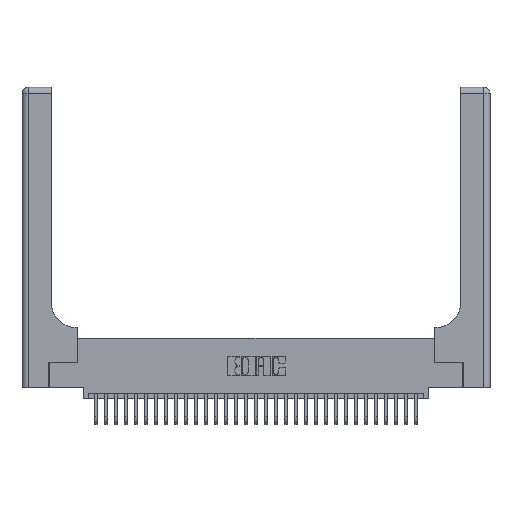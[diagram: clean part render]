
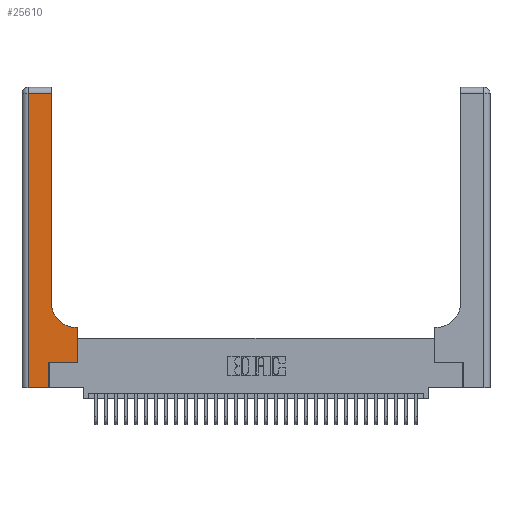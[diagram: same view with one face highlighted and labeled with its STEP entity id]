
A CAD part, top view. The second image highlights one B-rep face of the part: STEP entity #25610.
In plain terms, the highlighted planar face has unit normal (0, 0, 1).
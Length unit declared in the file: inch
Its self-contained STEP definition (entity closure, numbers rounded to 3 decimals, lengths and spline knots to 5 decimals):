
#931 = CARTESIAN_POINT ( 'NONE',  ( 0.269, 0.25, 0.37 ) ) ;
#1385 = VERTEX_POINT ( 'NONE', #3543 ) ;
#1602 = DIRECTION ( 'NONE',  ( 0., 1., 0. ) ) ;
#3370 = VECTOR ( 'NONE', #5774, 39.37008 ) ;
#3408 = CARTESIAN_POINT ( 'NONE',  ( 0.06, 3., 0.37 ) ) ;
#3427 = CARTESIAN_POINT ( 'NONE',  ( 0.06, 2.94, 0.37 ) ) ;
#3543 = CARTESIAN_POINT ( 'NONE',  ( 0.06, 0., 0.37 ) ) ;
#4092 = CARTESIAN_POINT ( 'NONE',  ( 0., 2.94, 0.37 ) ) ;
#4132 = LINE ( 'NONE', #20401, #3370 ) ;
#4817 = DIRECTION ( 'NONE',  ( 1., 0., 0. ) ) ;
#5692 = AXIS2_PLACEMENT_3D ( 'NONE', #26367, #11873, #28790 ) ;
#5774 = DIRECTION ( 'NONE',  ( 0., 1., 0. ) ) ;
#6044 = ORIENTED_EDGE ( 'NONE', *, *, #14439, .T. ) ;
#6551 = DIRECTION ( 'NONE',  ( -1., 0., 0. ) ) ;
#6573 = EDGE_CURVE ( 'NONE', #22003, #24052, #29202, .T. ) ;
#7005 = CARTESIAN_POINT ( 'NONE',  ( 0.5585, 0.6, 0.37 ) ) ;
#7516 = VECTOR ( 'NONE', #29604, 39.37008 ) ;
#8048 = DIRECTION ( 'NONE',  ( 0., 1., 0. ) ) ;
#8100 = VERTEX_POINT ( 'NONE', #19926 ) ;
#8304 = DIRECTION ( 'NONE',  ( 0., -1., 0. ) ) ;
#9020 = LINE ( 'NONE', #3408, #21969 ) ;
#9901 = VECTOR ( 'NONE', #1602, 39.37008 ) ;
#10525 = CARTESIAN_POINT ( 'NONE',  ( 0.5585, 0.25, 0.37 ) ) ;
#10785 = CARTESIAN_POINT ( 'NONE',  ( 0.269, 0., 0.37 ) ) ;
#10957 = CARTESIAN_POINT ( 'NONE',  ( 0.269, 0.25, 0.37 ) ) ;
#11873 = DIRECTION ( 'NONE',  ( 0., 0., -1. ) ) ;
#11879 = EDGE_CURVE ( 'NONE', #13759, #14379, #16385, .T. ) ;
#12665 = VERTEX_POINT ( 'NONE', #18512 ) ;
#13035 = EDGE_LOOP ( 'NONE', ( #22670, #28692, #20852, #26522, #20916, #6044, #26959, #21702, #21327 ) ) ;
#13418 = DIRECTION ( 'NONE',  ( 1., 0., 0. ) ) ;
#13748 = EDGE_CURVE ( 'NONE', #24052, #1385, #9020, .T. ) ;
#13759 = VERTEX_POINT ( 'NONE', #10785 ) ;
#14373 = CARTESIAN_POINT ( 'NONE',  ( 0.5415, 0.85, 0.37 ) ) ;
#14379 = VERTEX_POINT ( 'NONE', #931 ) ;
#14439 = EDGE_CURVE ( 'NONE', #14379, #8100, #16976, .T. ) ;
#14623 = FACE_OUTER_BOUND ( 'NONE', #13035, .T. ) ;
#15553 = AXIS2_PLACEMENT_3D ( 'NONE', #14373, #31276, #16799 ) ;
#16237 = VECTOR ( 'NONE', #13418, 39.37008 ) ;
#16363 = VECTOR ( 'NONE', #6551, 39.37008 ) ;
#16385 = LINE ( 'NONE', #30563, #9901 ) ;
#16765 = LINE ( 'NONE', #10525, #27376 ) ;
#16799 = DIRECTION ( 'NONE',  ( 1., 0., 0. ) ) ;
#16976 = LINE ( 'NONE', #10957, #16237 ) ;
#17472 = CARTESIAN_POINT ( 'NONE',  ( 0.2915, 0.6, 0.37 ) ) ;
#18281 = LINE ( 'NONE', #31456, #23933 ) ;
#18512 = CARTESIAN_POINT ( 'NONE',  ( 0.5415, 0.6, 0.37 ) ) ;
#18712 = VERTEX_POINT ( 'NONE', #7005 ) ;
#19237 = EDGE_CURVE ( 'NONE', #12665, #19729, #22366, .T. ) ;
#19729 = VERTEX_POINT ( 'NONE', #23460 ) ;
#19926 = CARTESIAN_POINT ( 'NONE',  ( 0.5585, 0.25, 0.37 ) ) ;
#20401 = CARTESIAN_POINT ( 'NONE',  ( 0.2915, 3., 0.37 ) ) ;
#20852 = ORIENTED_EDGE ( 'NONE', *, *, #13748, .T. ) ;
#20916 = ORIENTED_EDGE ( 'NONE', *, *, #11879, .T. ) ;
#21327 = ORIENTED_EDGE ( 'NONE', *, *, #19237, .T. ) ;
#21536 = PLANE ( 'NONE',  #5692 ) ;
#21702 = ORIENTED_EDGE ( 'NONE', *, *, #22936, .T. ) ;
#21755 = EDGE_CURVE ( 'NONE', #8100, #18712, #16765, .T. ) ;
#21969 = VECTOR ( 'NONE', #8304, 39.37008 ) ;
#22003 = VERTEX_POINT ( 'NONE', #28608 ) ;
#22106 = EDGE_CURVE ( 'NONE', #1385, #13759, #18281, .T. ) ;
#22366 = CIRCLE ( 'NONE', #15553, 0.25 ) ;
#22383 = EDGE_CURVE ( 'NONE', #19729, #22003, #4132, .T. ) ;
#22670 = ORIENTED_EDGE ( 'NONE', *, *, #22383, .T. ) ;
#22936 = EDGE_CURVE ( 'NONE', #18712, #12665, #27684, .T. ) ;
#23460 = CARTESIAN_POINT ( 'NONE',  ( 0.2915, 0.85, 0.37 ) ) ;
#23933 = VECTOR ( 'NONE', #4817, 39.37008 ) ;
#24052 = VERTEX_POINT ( 'NONE', #3427 ) ;
#25610 = ADVANCED_FACE ( 'NONE', ( #14623 ), #21536, .F. ) ;
#26367 = CARTESIAN_POINT ( 'NONE',  ( 0., 3., 0.37 ) ) ;
#26522 = ORIENTED_EDGE ( 'NONE', *, *, #22106, .T. ) ;
#26959 = ORIENTED_EDGE ( 'NONE', *, *, #21755, .T. ) ;
#27376 = VECTOR ( 'NONE', #8048, 39.37008 ) ;
#27684 = LINE ( 'NONE', #17472, #7516 ) ;
#28608 = CARTESIAN_POINT ( 'NONE',  ( 0.2915, 2.94, 0.37 ) ) ;
#28692 = ORIENTED_EDGE ( 'NONE', *, *, #6573, .T. ) ;
#28790 = DIRECTION ( 'NONE',  ( -1., 0., 0. ) ) ;
#29202 = LINE ( 'NONE', #4092, #16363 ) ;
#29604 = DIRECTION ( 'NONE',  ( -1., 0., 0. ) ) ;
#30563 = CARTESIAN_POINT ( 'NONE',  ( 0.269, 0., 0.37 ) ) ;
#31276 = DIRECTION ( 'NONE',  ( 0., 0., -1. ) ) ;
#31456 = CARTESIAN_POINT ( 'NONE',  ( 0., 0., 0.37 ) ) ;
